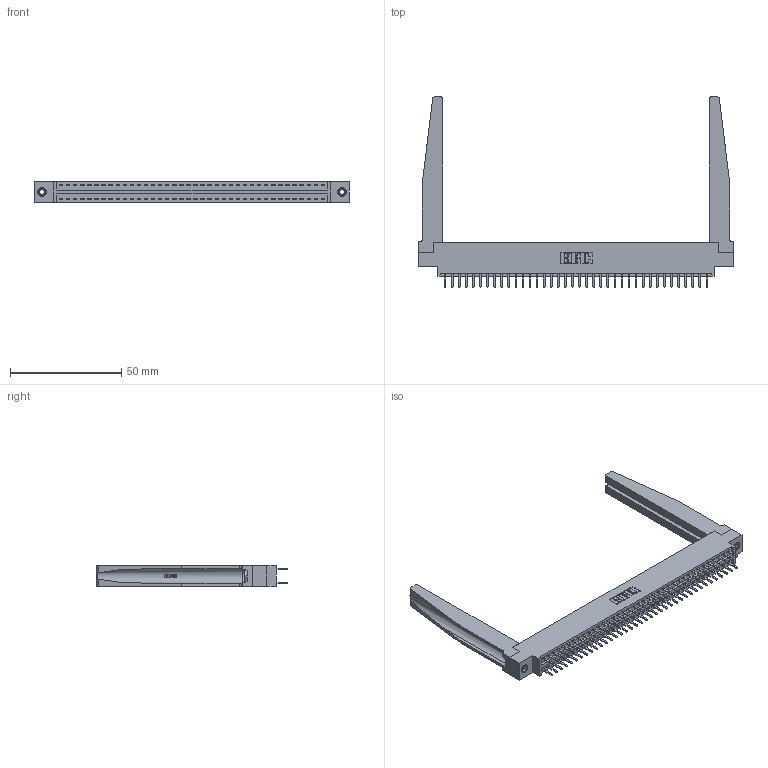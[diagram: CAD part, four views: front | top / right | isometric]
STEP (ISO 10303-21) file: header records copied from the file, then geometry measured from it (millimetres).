
FILE_DESCRIPTION (( 'STEP AP203' ), '1' );
FILE_NAME ('396-076-520-878.STEP', '2019-11-02T12:51:38', ( '' ), ( '' ), 'SwSTEP 2.0', 'SolidWorks 2016', '' );
FILE_SCHEMA (( 'CONFIG_CONTROL_DESIGN' ));
Length unit declared in the file: inch
Products named in the file (5): 346 Part_0.170 Offset - 0.156 Dia-TH; 345-292-001_345-293-120; 346-220-078_345-220-078; 345-250-001_345-250-001-102; 396-076-520-878
Assembly tree (81 placements, depth 2):
  396-076-520-878
    346 Part_0.170 Offset - 0.156 Dia-TH
    345-292-001_345-293-120  x76
    346-220-078_345-220-078  x2
    345-250-001_345-250-001-102  x2
Bounding box: 141.22 x 85.29 x 9.4 mm (x, y, z)
Volume: 20460.9 mm3; surface area: 25204.1 mm2
Topology: 81 solids, 81 shells, 4616 faces, 13337 edges, 8678 vertices
Faces by surface type: plane 3034, cylinder 1530, bspline 36, cone 12, torus 4
Entity records: 30332 total; most frequent: CARTESIAN_POINT 5955, ORIENTED_EDGE 4766, DIRECTION 4273, EDGE_CURVE 2383, VECTOR 2001, LINE 2001, VERTEX_POINT 1580, AXIS2_PLACEMENT_3D 1136
